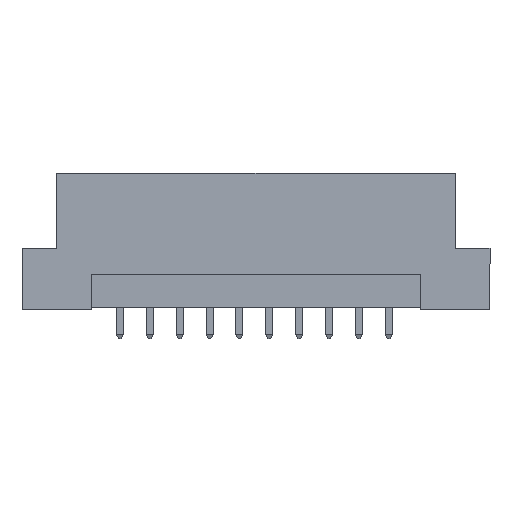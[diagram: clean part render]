
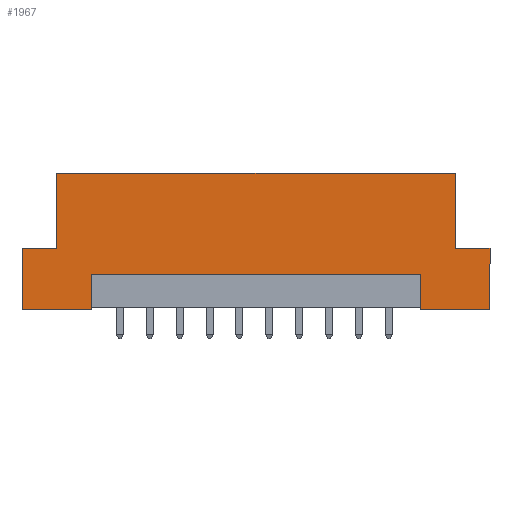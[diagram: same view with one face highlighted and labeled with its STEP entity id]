
A CAD part, front view. The second image highlights one B-rep face of the part: STEP entity #1967.
In plain terms, the highlighted planar face has unit normal (0, -1, 0).
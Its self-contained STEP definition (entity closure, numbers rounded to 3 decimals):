
#195 = VECTOR ( 'NONE', #3142, 1000. ) ;
#218 = DIRECTION ( 'NONE',  ( 0., 0., -1. ) ) ;
#219 = VERTEX_POINT ( 'NONE', #1765 ) ;
#221 = CARTESIAN_POINT ( 'NONE',  ( 14., -4.3, 3. ) ) ;
#231 = PLANE ( 'NONE',  #3391 ) ;
#255 = ORIENTED_EDGE ( 'NONE', *, *, #5357, .F. ) ;
#320 = CARTESIAN_POINT ( 'NONE',  ( -14., -4.3, 3. ) ) ;
#426 = EDGE_CURVE ( 'NONE', #2382, #219, #1674, .T. ) ;
#487 = LINE ( 'NONE', #2580, #3911 ) ;
#534 = CARTESIAN_POINT ( 'NONE',  ( 16.94, -4.3, 5.2 ) ) ;
#643 = ORIENTED_EDGE ( 'NONE', *, *, #2872, .F. ) ;
#647 = FACE_OUTER_BOUND ( 'NONE', #4096, .T. ) ;
#680 = VERTEX_POINT ( 'NONE', #1816 ) ;
#724 = DIRECTION ( 'NONE',  ( 1., 0., 0. ) ) ;
#789 = LINE ( 'NONE', #1231, #1900 ) ;
#794 = ORIENTED_EDGE ( 'NONE', *, *, #1846, .F. ) ;
#987 = EDGE_CURVE ( 'NONE', #1897, #2107, #3398, .T. ) ;
#1168 = DIRECTION ( 'NONE',  ( 1., 0., 0. ) ) ;
#1231 = CARTESIAN_POINT ( 'NONE',  ( 14., -4.3, 0.2 ) ) ;
#1276 = VECTOR ( 'NONE', #4369, 1000. ) ;
#1296 = CARTESIAN_POINT ( 'NONE',  ( 19.9, -4.3, 0. ) ) ;
#1327 = ORIENTED_EDGE ( 'NONE', *, *, #1482, .F. ) ;
#1340 = EDGE_CURVE ( 'NONE', #3394, #219, #3089, .T. ) ;
#1482 = EDGE_CURVE ( 'NONE', #3372, #2107, #487, .T. ) ;
#1674 = LINE ( 'NONE', #2142, #1714 ) ;
#1714 = VECTOR ( 'NONE', #4251, 1000. ) ;
#1765 = CARTESIAN_POINT ( 'NONE',  ( 19.9, -4.3, 0. ) ) ;
#1807 = LINE ( 'NONE', #4788, #195 ) ;
#1816 = CARTESIAN_POINT ( 'NONE',  ( -16.94, -4.3, 5.2 ) ) ;
#1846 = EDGE_CURVE ( 'NONE', #3193, #2382, #3776, .T. ) ;
#1897 = VERTEX_POINT ( 'NONE', #2775 ) ;
#1900 = VECTOR ( 'NONE', #5050, 1000. ) ;
#1949 = CARTESIAN_POINT ( 'NONE',  ( -16.94, -4.3, 5.2 ) ) ;
#1967 = ADVANCED_FACE ( 'NONE', ( #647 ), #231, .F. ) ;
#2057 = VECTOR ( 'NONE', #218, 1000. ) ;
#2107 = VERTEX_POINT ( 'NONE', #4241 ) ;
#2124 = CARTESIAN_POINT ( 'NONE',  ( 19.9, -4.3, 5.2 ) ) ;
#2142 = CARTESIAN_POINT ( 'NONE',  ( 19.9, -4.3, 11.6 ) ) ;
#2191 = EDGE_CURVE ( 'NONE', #3372, #4471, #2349, .T. ) ;
#2340 = VECTOR ( 'NONE', #3422, 1000. ) ;
#2349 = LINE ( 'NONE', #4018, #4071 ) ;
#2382 = VERTEX_POINT ( 'NONE', #2124 ) ;
#2403 = VECTOR ( 'NONE', #4692, 1000. ) ;
#2448 = EDGE_CURVE ( 'NONE', #4187, #1897, #4487, .T. ) ;
#2580 = CARTESIAN_POINT ( 'NONE',  ( -14., -4.3, 0.2 ) ) ;
#2684 = EDGE_CURVE ( 'NONE', #4187, #680, #1807, .T. ) ;
#2705 = CARTESIAN_POINT ( 'NONE',  ( 19.9, -4.3, 0. ) ) ;
#2712 = ORIENTED_EDGE ( 'NONE', *, *, #2448, .T. ) ;
#2775 = CARTESIAN_POINT ( 'NONE',  ( -19.9, -4.3, 0. ) ) ;
#2861 = EDGE_CURVE ( 'NONE', #4379, #5404, #5319, .T. ) ;
#2871 = CARTESIAN_POINT ( 'NONE',  ( 19.9, -4.3, 11.6 ) ) ;
#2872 = EDGE_CURVE ( 'NONE', #680, #4379, #3315, .T. ) ;
#3081 = CARTESIAN_POINT ( 'NONE',  ( 16.94, -4.3, 5.2 ) ) ;
#3089 = LINE ( 'NONE', #2705, #1276 ) ;
#3142 = DIRECTION ( 'NONE',  ( 1., 0., 0. ) ) ;
#3193 = VERTEX_POINT ( 'NONE', #3081 ) ;
#3197 = CARTESIAN_POINT ( 'NONE',  ( -19.9, -4.3, 11.6 ) ) ;
#3252 = ORIENTED_EDGE ( 'NONE', *, *, #987, .T. ) ;
#3255 = DIRECTION ( 'NONE',  ( 0., 0., 1. ) ) ;
#3315 = LINE ( 'NONE', #1949, #4862 ) ;
#3344 = ORIENTED_EDGE ( 'NONE', *, *, #2191, .T. ) ;
#3372 = VERTEX_POINT ( 'NONE', #320 ) ;
#3391 = AXIS2_PLACEMENT_3D ( 'NONE', #5302, #4887, #5361 ) ;
#3394 = VERTEX_POINT ( 'NONE', #5367 ) ;
#3398 = LINE ( 'NONE', #1296, #2340 ) ;
#3422 = DIRECTION ( 'NONE',  ( 1., 0., 0. ) ) ;
#3521 = ORIENTED_EDGE ( 'NONE', *, *, #3597, .T. ) ;
#3597 = EDGE_CURVE ( 'NONE', #3193, #5404, #4327, .T. ) ;
#3665 = ORIENTED_EDGE ( 'NONE', *, *, #2861, .F. ) ;
#3776 = LINE ( 'NONE', #5013, #4707 ) ;
#3911 = VECTOR ( 'NONE', #4248, 1000. ) ;
#4018 = CARTESIAN_POINT ( 'NONE',  ( -14., -4.3, 3. ) ) ;
#4071 = VECTOR ( 'NONE', #4765, 1000. ) ;
#4096 = EDGE_LOOP ( 'NONE', ( #3344, #255, #4301, #4952, #794, #3521, #3665, #643, #4845, #2712, #3252, #1327 ) ) ;
#4139 = CARTESIAN_POINT ( 'NONE',  ( 16.94, -4.3, 11.6 ) ) ;
#4187 = VERTEX_POINT ( 'NONE', #5108 ) ;
#4241 = CARTESIAN_POINT ( 'NONE',  ( -14., -4.3, 0. ) ) ;
#4248 = DIRECTION ( 'NONE',  ( 0., 0., -1. ) ) ;
#4251 = DIRECTION ( 'NONE',  ( 0., 0., -1. ) ) ;
#4301 = ORIENTED_EDGE ( 'NONE', *, *, #1340, .T. ) ;
#4327 = LINE ( 'NONE', #534, #2403 ) ;
#4369 = DIRECTION ( 'NONE',  ( 1., 0., 0. ) ) ;
#4379 = VERTEX_POINT ( 'NONE', #4458 ) ;
#4458 = CARTESIAN_POINT ( 'NONE',  ( -16.94, -4.3, 11.6 ) ) ;
#4471 = VERTEX_POINT ( 'NONE', #221 ) ;
#4487 = LINE ( 'NONE', #3197, #2057 ) ;
#4513 = VECTOR ( 'NONE', #1168, 1000. ) ;
#4692 = DIRECTION ( 'NONE',  ( 0., 0., 1. ) ) ;
#4707 = VECTOR ( 'NONE', #724, 1000. ) ;
#4765 = DIRECTION ( 'NONE',  ( 1., 0., 0. ) ) ;
#4788 = CARTESIAN_POINT ( 'NONE',  ( -19.9, -4.3, 5.2 ) ) ;
#4845 = ORIENTED_EDGE ( 'NONE', *, *, #2684, .F. ) ;
#4862 = VECTOR ( 'NONE', #3255, 1000. ) ;
#4887 = DIRECTION ( 'NONE',  ( 0., 1., 0. ) ) ;
#4952 = ORIENTED_EDGE ( 'NONE', *, *, #426, .F. ) ;
#5013 = CARTESIAN_POINT ( 'NONE',  ( 19.9, -4.3, 5.2 ) ) ;
#5050 = DIRECTION ( 'NONE',  ( 0., 0., 1. ) ) ;
#5108 = CARTESIAN_POINT ( 'NONE',  ( -19.9, -4.3, 5.2 ) ) ;
#5302 = CARTESIAN_POINT ( 'NONE',  ( 19.9, -4.3, 11.6 ) ) ;
#5319 = LINE ( 'NONE', #2871, #4513 ) ;
#5357 = EDGE_CURVE ( 'NONE', #3394, #4471, #789, .T. ) ;
#5361 = DIRECTION ( 'NONE',  ( -1., 0., 0. ) ) ;
#5367 = CARTESIAN_POINT ( 'NONE',  ( 14., -4.3, 0. ) ) ;
#5404 = VERTEX_POINT ( 'NONE', #4139 ) ;
